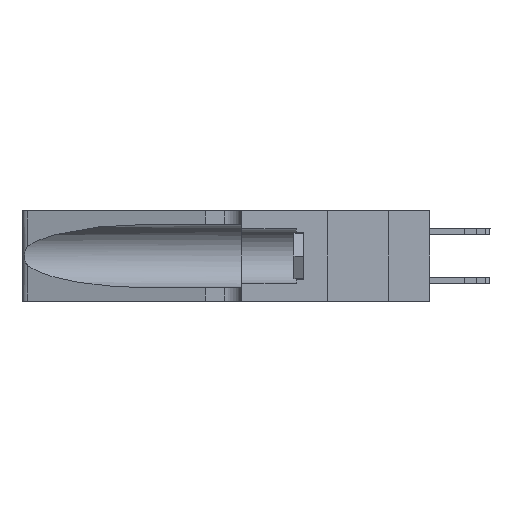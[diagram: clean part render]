
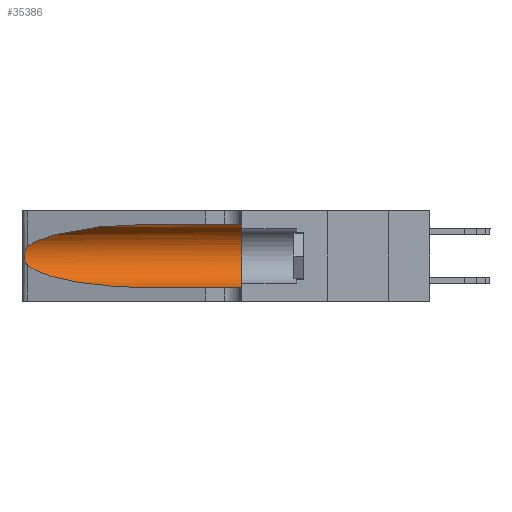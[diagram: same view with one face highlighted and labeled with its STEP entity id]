
A CAD part, left-side view. The second image highlights one B-rep face of the part: STEP entity #35386.
In plain terms, the highlighted cylindrical face has radius 3.308 mm (diameter 6.617 mm), a partial arc.
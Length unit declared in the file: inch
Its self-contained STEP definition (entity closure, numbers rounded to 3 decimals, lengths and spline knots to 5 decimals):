
#905 = CYLINDRICAL_SURFACE ( 'NONE', #23698, 0.13025 ) ;
#1358 = ORIENTED_EDGE ( 'NONE', *, *, #34297, .T. ) ;
#1916 = CARTESIAN_POINT ( 'NONE',  ( 0.25487, 1.22718, 0.14631 ) ) ;
#2129 = CARTESIAN_POINT ( 'NONE',  ( 0.1305, 1.61858, 0.05475 ) ) ;
#2178 = CARTESIAN_POINT ( 'NONE',  ( 0.25854, 1.2359, 0.20912 ) ) ;
#2292 = DIRECTION ( 'NONE',  ( 0., 0., -1. ) ) ;
#2313 = CARTESIAN_POINT ( 'NONE',  ( 0.2373, 1.15595, 0.08982 ) ) ;
#2552 = CARTESIAN_POINT ( 'NONE',  ( 0.25639, 1.23186, 0.15144 ) ) ;
#3803 =( BOUNDED_CURVE ( )  B_SPLINE_CURVE ( 3, ( #1916, #2313, #17018, #22262 ),
 .UNSPECIFIED., .F., .T. ) 
 B_SPLINE_CURVE_WITH_KNOTS ( ( 4, 4 ),
 ( 3.44316, 4.71239 ),
 .UNSPECIFIED. ) 
 CURVE ( )  GEOMETRIC_REPRESENTATION_ITEM ( )  RATIONAL_B_SPLINE_CURVE ( ( 1., 0.87, 0.87, 1. ) ) 
 REPRESENTATION_ITEM ( '' )  );
#4012 = CARTESIAN_POINT ( 'NONE',  ( 0.1305, 0.35, 0.31525 ) ) ;
#4109 = FACE_OUTER_BOUND ( 'NONE', #26241, .T. ) ;
#5671 = CARTESIAN_POINT ( 'NONE',  ( 0.2373, 1.15595, 0.28018 ) ) ;
#5751 = ORIENTED_EDGE ( 'NONE', *, *, #12298, .T. ) ;
#7806 = CARTESIAN_POINT ( 'NONE',  ( 0.1305, 0.72297, 0.05475 ) ) ;
#7844 = ORIENTED_EDGE ( 'NONE', *, *, #37278, .F. ) ;
#8614 = CARTESIAN_POINT ( 'NONE',  ( 0.1305, 0.72297, 0.31525 ) ) ;
#8626 = VERTEX_POINT ( 'NONE', #13412 ) ;
#9791 = ORIENTED_EDGE ( 'NONE', *, *, #25703, .F. ) ;
#11247 = CARTESIAN_POINT ( 'NONE',  ( 0.26018, 1.23835, 0.19895 ) ) ;
#12234 = B_SPLINE_CURVE_WITH_KNOTS ( 'NONE', 3,
 ( #14202, #28706, #34296, #28573, #2178, #11247, #31467, #31606, #25895, #17139, #37519, #2552, #22993, #20201 ),
 .UNSPECIFIED., .F., .F.,
 ( 4, 2, 2, 2, 2, 2, 4 ),
 ( 0., 0.00027, 0.00053, 0.00107, 0.0016, 0.00187, 0.00214 ),
 .UNSPECIFIED. ) ;
#12298 = EDGE_CURVE ( 'NONE', #30974, #24746, #3803, .T. ) ;
#13412 = CARTESIAN_POINT ( 'NONE',  ( 0.1305, 0.35, 0.05475 ) ) ;
#13468 = CARTESIAN_POINT ( 'NONE',  ( 0.25487, 1.22718, 0.14631 ) ) ;
#14202 = CARTESIAN_POINT ( 'NONE',  ( 0.25487, 1.22718, 0.22369 ) ) ;
#14256 = LINE ( 'NONE', #32963, #23343 ) ;
#15097 = VERTEX_POINT ( 'NONE', #29859 ) ;
#15671 = AXIS2_PLACEMENT_3D ( 'NONE', #20297, #37481, #23215 ) ;
#16745 = CARTESIAN_POINT ( 'NONE',  ( 0.1305, 1.61858, 0.185 ) ) ;
#17018 = CARTESIAN_POINT ( 'NONE',  ( 0.18966, 0.96281, 0.05475 ) ) ;
#17139 = CARTESIAN_POINT ( 'NONE',  ( 0.25856, 1.23593, 0.16098 ) ) ;
#17323 = LINE ( 'NONE', #2129, #30921 ) ;
#18497 = DIRECTION ( 'NONE',  ( 0., -1., 0. ) ) ;
#18533 = ORIENTED_EDGE ( 'NONE', *, *, #22466, .T. ) ;
#20119 = CARTESIAN_POINT ( 'NONE',  ( 0.25487, 1.22718, 0.22369 ) ) ;
#20201 = CARTESIAN_POINT ( 'NONE',  ( 0.25487, 1.22718, 0.14631 ) ) ;
#20297 = CARTESIAN_POINT ( 'NONE',  ( 0.1305, 0.35, 0.185 ) ) ;
#21306 = DIRECTION ( 'NONE',  ( 0., -1., 0. ) ) ;
#22262 = CARTESIAN_POINT ( 'NONE',  ( 0.1305, 0.72297, 0.05475 ) ) ;
#22274 = EDGE_CURVE ( 'NONE', #24746, #8626, #17323, .T. ) ;
#22466 = EDGE_CURVE ( 'NONE', #27252, #30974, #12234, .T. ) ;
#22993 = CARTESIAN_POINT ( 'NONE',  ( 0.25555, 1.22993, 0.14849 ) ) ;
#23215 = DIRECTION ( 'NONE',  ( 0., 0., 1. ) ) ;
#23343 = VECTOR ( 'NONE', #21306, 39.37008 ) ;
#23698 = AXIS2_PLACEMENT_3D ( 'NONE', #16745, #28443, #2292 ) ;
#24746 = VERTEX_POINT ( 'NONE', #7806 ) ;
#25703 = EDGE_CURVE ( 'NONE', #34584, #8626, #34223, .T. ) ;
#25895 = CARTESIAN_POINT ( 'NONE',  ( 0.26017, 1.23833, 0.17102 ) ) ;
#26241 = EDGE_LOOP ( 'NONE', ( #1358, #18533, #5751, #35799, #9791, #7844 ) ) ;
#27252 = VERTEX_POINT ( 'NONE', #20119 ) ;
#28443 = DIRECTION ( 'NONE',  ( 0., -1., 0. ) ) ;
#28573 = CARTESIAN_POINT ( 'NONE',  ( 0.25787, 1.23484, 0.2124 ) ) ;
#28706 = CARTESIAN_POINT ( 'NONE',  ( 0.25555, 1.22994, 0.2215 ) ) ;
#28907 = CARTESIAN_POINT ( 'NONE',  ( 0.18966, 0.96281, 0.31525 ) ) ;
#29263 = CARTESIAN_POINT ( 'NONE',  ( 0.25487, 1.22718, 0.22369 ) ) ;
#29859 = CARTESIAN_POINT ( 'NONE',  ( 0.1305, 0.72297, 0.31525 ) ) ;
#30921 = VECTOR ( 'NONE', #18497, 39.37008 ) ;
#30974 = VERTEX_POINT ( 'NONE', #13468 ) ;
#31467 = CARTESIAN_POINT ( 'NONE',  ( 0.26075, 1.23896, 0.19203 ) ) ;
#31606 = CARTESIAN_POINT ( 'NONE',  ( 0.26075, 1.23896, 0.178 ) ) ;
#32963 = CARTESIAN_POINT ( 'NONE',  ( 0.1305, 1.61858, 0.31525 ) ) ;
#34223 = CIRCLE ( 'NONE', #15671, 0.13025 ) ;
#34296 = CARTESIAN_POINT ( 'NONE',  ( 0.25639, 1.23184, 0.21858 ) ) ;
#34297 = EDGE_CURVE ( 'NONE', #15097, #27252, #34897, .T. ) ;
#34584 = VERTEX_POINT ( 'NONE', #4012 ) ;
#34897 =( BOUNDED_CURVE ( )  B_SPLINE_CURVE ( 3, ( #8614, #28907, #5671, #29263 ),
 .UNSPECIFIED., .F., .F. ) 
 B_SPLINE_CURVE_WITH_KNOTS ( ( 4, 4 ),
 ( 1.5708, 2.84003 ),
 .UNSPECIFIED. ) 
 CURVE ( )  GEOMETRIC_REPRESENTATION_ITEM ( )  RATIONAL_B_SPLINE_CURVE ( ( 1., 0.87, 0.87, 1. ) ) 
 REPRESENTATION_ITEM ( '' )  );
#35386 = ADVANCED_FACE ( 'NONE', ( #4109 ), #905, .F. ) ;
#35799 = ORIENTED_EDGE ( 'NONE', *, *, #22274, .T. ) ;
#37278 = EDGE_CURVE ( 'NONE', #15097, #34584, #14256, .T. ) ;
#37481 = DIRECTION ( 'NONE',  ( 0., 1., 0. ) ) ;
#37519 = CARTESIAN_POINT ( 'NONE',  ( 0.25789, 1.23486, 0.15765 ) ) ;
